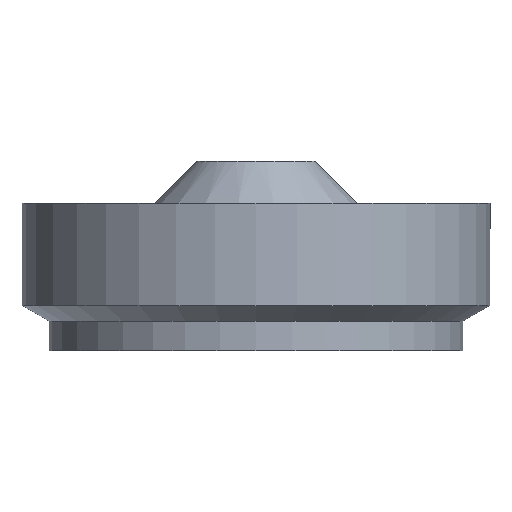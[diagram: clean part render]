
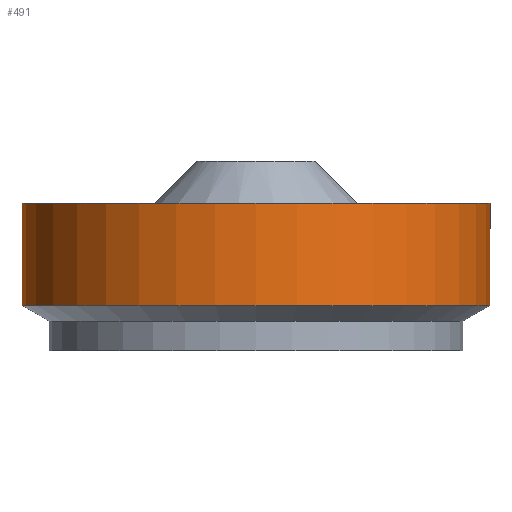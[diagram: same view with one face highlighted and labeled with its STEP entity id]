
A CAD part, left-side view. The second image highlights one B-rep face of the part: STEP entity #491.
In plain terms, the highlighted cylindrical face has radius 25.146 mm (diameter 50.292 mm), a partial arc.
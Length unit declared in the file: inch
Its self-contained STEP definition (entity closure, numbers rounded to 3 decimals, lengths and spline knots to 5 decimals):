
#5 = DIRECTION ( 'NONE',  ( 0., 0., -1. ) ) ;
#89 = CIRCLE ( 'NONE', #364, 0.99 ) ;
#95 = EDGE_LOOP ( 'NONE', ( #425, #146, #589, #553 ) ) ;
#126 = EDGE_CURVE ( 'NONE', #569, #137, #704, .T. ) ;
#137 = VERTEX_POINT ( 'NONE', #625 ) ;
#140 = DIRECTION ( 'NONE',  ( 0., 0., -1. ) ) ;
#146 = ORIENTED_EDGE ( 'NONE', *, *, #169, .T. ) ;
#154 = DIRECTION ( 'NONE',  ( 0., 0., -1. ) ) ;
#156 = CYLINDRICAL_SURFACE ( 'NONE', #341, 0.99 ) ;
#169 = EDGE_CURVE ( 'NONE', #361, #569, #329, .T. ) ;
#257 = CARTESIAN_POINT ( 'NONE',  ( 0., 0.99, 0.625 ) ) ;
#271 = DIRECTION ( 'NONE',  ( 0., 0., -1. ) ) ;
#316 = FACE_OUTER_BOUND ( 'NONE', #95, .T. ) ;
#329 = CIRCLE ( 'NONE', #433, 0.99 ) ;
#341 = AXIS2_PLACEMENT_3D ( 'NONE', #600, #154, #543 ) ;
#361 = VERTEX_POINT ( 'NONE', #528 ) ;
#364 = AXIS2_PLACEMENT_3D ( 'NONE', #665, #271, #560 ) ;
#385 = LINE ( 'NONE', #514, #660 ) ;
#387 = CARTESIAN_POINT ( 'NONE',  ( 0., 0., 0.625 ) ) ;
#388 = DIRECTION ( 'NONE',  ( 0., 1., 0. ) ) ;
#425 = ORIENTED_EDGE ( 'NONE', *, *, #694, .F. ) ;
#433 = AXIS2_PLACEMENT_3D ( 'NONE', #387, #5, #388 ) ;
#463 = VERTEX_POINT ( 'NONE', #703 ) ;
#490 = DIRECTION ( 'NONE',  ( 0., 0., -1. ) ) ;
#491 = ADVANCED_FACE ( 'NONE', ( #316 ), #156, .T. ) ;
#514 = CARTESIAN_POINT ( 'NONE',  ( 0., -0.99, 0. ) ) ;
#528 = CARTESIAN_POINT ( 'NONE',  ( 0., -0.99, 0.625 ) ) ;
#543 = DIRECTION ( 'NONE',  ( 0., 1., 0. ) ) ;
#546 = VECTOR ( 'NONE', #490, 39.37008 ) ;
#553 = ORIENTED_EDGE ( 'NONE', *, *, #626, .F. ) ;
#557 = CARTESIAN_POINT ( 'NONE',  ( 0., 0.99, 0. ) ) ;
#560 = DIRECTION ( 'NONE',  ( 0., 1., 0. ) ) ;
#569 = VERTEX_POINT ( 'NONE', #257 ) ;
#589 = ORIENTED_EDGE ( 'NONE', *, *, #126, .T. ) ;
#600 = CARTESIAN_POINT ( 'NONE',  ( 0., 0., 0. ) ) ;
#625 = CARTESIAN_POINT ( 'NONE',  ( 0., 0.99, 0.1914 ) ) ;
#626 = EDGE_CURVE ( 'NONE', #463, #137, #89, .T. ) ;
#660 = VECTOR ( 'NONE', #140, 39.37008 ) ;
#665 = CARTESIAN_POINT ( 'NONE',  ( 0., 0., 0.1914 ) ) ;
#694 = EDGE_CURVE ( 'NONE', #361, #463, #385, .T. ) ;
#703 = CARTESIAN_POINT ( 'NONE',  ( 0., -0.99, 0.1914 ) ) ;
#704 = LINE ( 'NONE', #557, #546 ) ;
